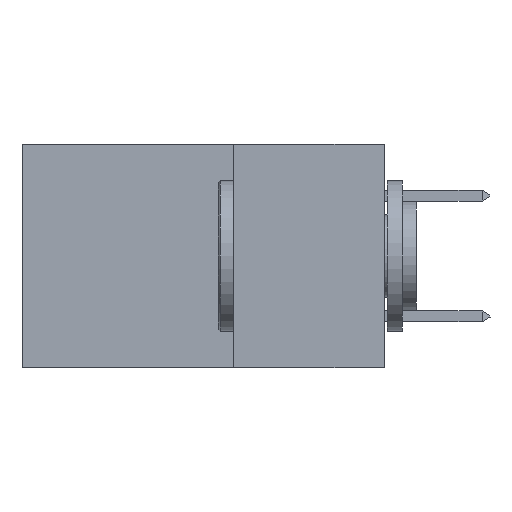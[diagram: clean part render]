
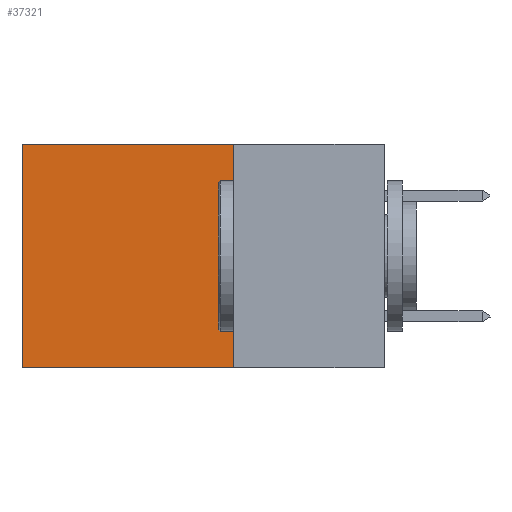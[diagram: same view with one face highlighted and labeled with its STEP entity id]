
A CAD part, left-side view. The second image highlights one B-rep face of the part: STEP entity #37321.
In plain terms, the highlighted planar face has unit normal (-1, 0, 0).
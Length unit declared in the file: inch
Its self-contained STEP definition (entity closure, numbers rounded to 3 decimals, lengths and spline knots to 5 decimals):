
#267 = ORIENTED_EDGE ( 'NONE', *, *, #40108, .T. ) ;
#1569 = CARTESIAN_POINT ( 'NONE',  ( 0.2875, 0.25, 0. ) ) ;
#2669 = CARTESIAN_POINT ( 'NONE',  ( 0.2875, 0.6, 0. ) ) ;
#4808 = DIRECTION ( 'NONE',  ( 0., 0., -1. ) ) ;
#5967 = VECTOR ( 'NONE', #25264, 39.37008 ) ;
#6544 = LINE ( 'NONE', #6700, #38511 ) ;
#6700 = CARTESIAN_POINT ( 'NONE',  ( 0.2875, 0.6, 0. ) ) ;
#10177 = CARTESIAN_POINT ( 'NONE',  ( 0.2875, 0.25, -0.37 ) ) ;
#10984 = VECTOR ( 'NONE', #38060, 39.37008 ) ;
#12717 = EDGE_CURVE ( 'NONE', #36180, #19546, #30752, .T. ) ;
#14760 = CARTESIAN_POINT ( 'NONE',  ( 0.2875, 0.25, -0.37 ) ) ;
#18219 = VERTEX_POINT ( 'NONE', #26834 ) ;
#18472 = VECTOR ( 'NONE', #26356, 39.37008 ) ;
#19457 = LINE ( 'NONE', #23267, #18472 ) ;
#19546 = VERTEX_POINT ( 'NONE', #14760 ) ;
#22348 = EDGE_CURVE ( 'NONE', #36180, #31642, #19457, .T. ) ;
#23232 = ORIENTED_EDGE ( 'NONE', *, *, #24138, .F. ) ;
#23267 = CARTESIAN_POINT ( 'NONE',  ( 0.2875, 0.25, 0. ) ) ;
#23510 = DIRECTION ( 'NONE',  ( 1., 0., 0. ) ) ;
#24138 = EDGE_CURVE ( 'NONE', #19546, #18219, #29480, .T. ) ;
#25264 = DIRECTION ( 'NONE',  ( 0., 0., -1. ) ) ;
#25301 = EDGE_LOOP ( 'NONE', ( #267, #23232, #26831, #30409 ) ) ;
#26356 = DIRECTION ( 'NONE',  ( 0., 1., 0. ) ) ;
#26831 = ORIENTED_EDGE ( 'NONE', *, *, #12717, .F. ) ;
#26834 = CARTESIAN_POINT ( 'NONE',  ( 0.2875, 0.6, -0.37 ) ) ;
#29480 = LINE ( 'NONE', #10177, #10984 ) ;
#30409 = ORIENTED_EDGE ( 'NONE', *, *, #22348, .T. ) ;
#30752 = LINE ( 'NONE', #34526, #5967 ) ;
#31526 = DIRECTION ( 'NONE',  ( 0., 0., -1. ) ) ;
#31642 = VERTEX_POINT ( 'NONE', #2669 ) ;
#32653 = PLANE ( 'NONE',  #40004 ) ;
#32749 = FACE_OUTER_BOUND ( 'NONE', #25301, .T. ) ;
#33526 = CARTESIAN_POINT ( 'NONE',  ( 0.2875, 0.25, 0. ) ) ;
#34526 = CARTESIAN_POINT ( 'NONE',  ( 0.2875, 0.25, 0. ) ) ;
#36180 = VERTEX_POINT ( 'NONE', #33526 ) ;
#37321 = ADVANCED_FACE ( 'NONE', ( #32749 ), #32653, .F. ) ;
#38060 = DIRECTION ( 'NONE',  ( 0., 1., 0. ) ) ;
#38511 = VECTOR ( 'NONE', #31526, 39.37008 ) ;
#40004 = AXIS2_PLACEMENT_3D ( 'NONE', #1569, #23510, #4808 ) ;
#40108 = EDGE_CURVE ( 'NONE', #31642, #18219, #6544, .T. ) ;
